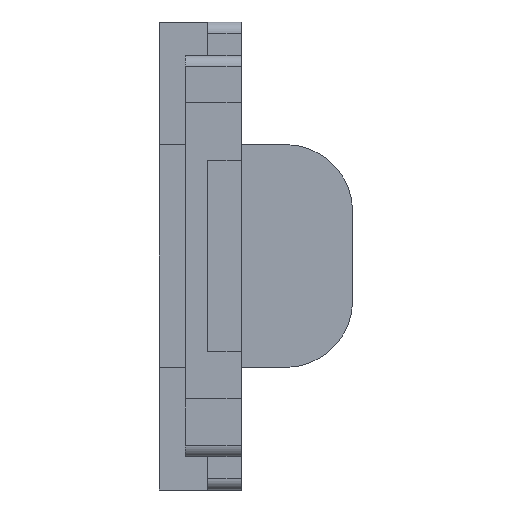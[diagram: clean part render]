
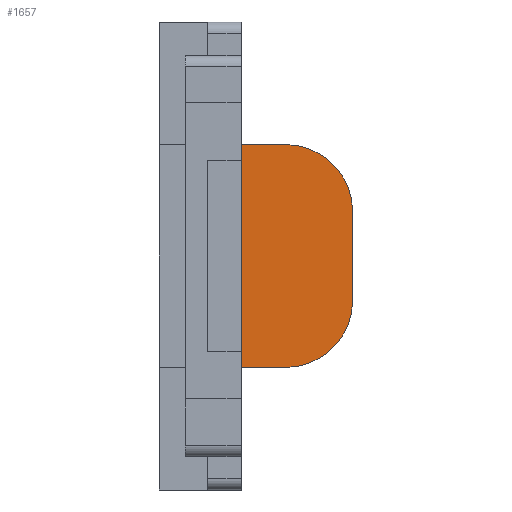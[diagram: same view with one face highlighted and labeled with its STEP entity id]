
A CAD part, front view. The second image highlights one B-rep face of the part: STEP entity #1657.
In plain terms, the highlighted planar face has unit normal (0, -1, 0).
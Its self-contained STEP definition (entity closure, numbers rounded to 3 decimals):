
#162 = PLANE('',#163);
#163 = AXIS2_PLACEMENT_3D('',#164,#165,#166);
#164 = CARTESIAN_POINT('',(8.,-4.,20.));
#165 = DIRECTION('',(1.,0.,0.));
#166 = DIRECTION('',(0.,0.,-1.));
#179 = VERTEX_POINT('',#180);
#180 = CARTESIAN_POINT('',(8.,-4.,20.));
#514 = PLANE('',#515);
#515 = AXIS2_PLACEMENT_3D('',#516,#517,#518);
#516 = CARTESIAN_POINT('',(0.,0.,20.));
#517 = DIRECTION('',(0.,0.,1.));
#518 = DIRECTION('',(1.,0.,0.));
#795 = VERTEX_POINT('',#796);
#796 = CARTESIAN_POINT('',(8.,-4.,0.));
#817 = EDGE_CURVE('',#795,#179,#818,.T.);
#818 = SURFACE_CURVE('',#819,(#823,#830),.PCURVE_S1.);
#819 = LINE('',#820,#821);
#820 = CARTESIAN_POINT('',(8.,-4.,-11.));
#821 = VECTOR('',#822,1.);
#822 = DIRECTION('',(0.,0.,1.));
#823 = PCURVE('',#162,#824);
#824 = DEFINITIONAL_REPRESENTATION('',(#825),#829);
#825 = LINE('',#826,#827);
#826 = CARTESIAN_POINT('',(31.,0.));
#827 = VECTOR('',#828,1.);
#828 = DIRECTION('',(-1.,0.));
#829 = ( GEOMETRIC_REPRESENTATION_CONTEXT(2) 
PARAMETRIC_REPRESENTATION_CONTEXT() REPRESENTATION_CONTEXT('2D SPACE',''
  ) );
#830 = PCURVE('',#831,#836);
#831 = PLANE('',#832);
#832 = AXIS2_PLACEMENT_3D('',#833,#834,#835);
#833 = CARTESIAN_POINT('',(3.,-4.,20.));
#834 = DIRECTION('',(0.,-1.,0.));
#835 = DIRECTION('',(1.,0.,0.));
#836 = DEFINITIONAL_REPRESENTATION('',(#837),#841);
#837 = LINE('',#838,#839);
#838 = CARTESIAN_POINT('',(5.,-31.));
#839 = VECTOR('',#840,1.);
#840 = DIRECTION('',(0.,1.));
#841 = ( GEOMETRIC_REPRESENTATION_CONTEXT(2) 
PARAMETRIC_REPRESENTATION_CONTEXT() REPRESENTATION_CONTEXT('2D SPACE',''
  ) );
#1479 = VERTEX_POINT('',#1480);
#1480 = CARTESIAN_POINT('',(12.,-4.,20.));
#1494 = CYLINDRICAL_SURFACE('',#1495,6.);
#1495 = AXIS2_PLACEMENT_3D('',#1496,#1497,#1498);
#1496 = CARTESIAN_POINT('',(12.,0.,14.));
#1497 = DIRECTION('',(0.,-1.,0.));
#1498 = DIRECTION('',(1.,0.,0.));
#1560 = EDGE_CURVE('',#179,#1479,#1561,.T.);
#1561 = SURFACE_CURVE('',#1562,(#1566,#1573),.PCURVE_S1.);
#1562 = LINE('',#1563,#1564);
#1563 = CARTESIAN_POINT('',(3.,-4.,20.));
#1564 = VECTOR('',#1565,1.);
#1565 = DIRECTION('',(1.,0.,0.));
#1566 = PCURVE('',#514,#1567);
#1567 = DEFINITIONAL_REPRESENTATION('',(#1568),#1572);
#1568 = LINE('',#1569,#1570);
#1569 = CARTESIAN_POINT('',(3.,-4.));
#1570 = VECTOR('',#1571,1.);
#1571 = DIRECTION('',(1.,0.));
#1572 = ( GEOMETRIC_REPRESENTATION_CONTEXT(2) 
PARAMETRIC_REPRESENTATION_CONTEXT() REPRESENTATION_CONTEXT('2D SPACE',''
  ) );
#1573 = PCURVE('',#831,#1574);
#1574 = DEFINITIONAL_REPRESENTATION('',(#1575),#1579);
#1575 = LINE('',#1576,#1577);
#1576 = CARTESIAN_POINT('',(0.,0.));
#1577 = VECTOR('',#1578,1.);
#1578 = DIRECTION('',(1.,0.));
#1579 = ( GEOMETRIC_REPRESENTATION_CONTEXT(2) 
PARAMETRIC_REPRESENTATION_CONTEXT() REPRESENTATION_CONTEXT('2D SPACE',''
  ) );
#1657 = ADVANCED_FACE('',(#1658),#831,.T.);
#1658 = FACE_BOUND('',#1659,.T.);
#1659 = EDGE_LOOP('',(#1660,#1695,#1721,#1743,#1744,#1745));
#1660 = ORIENTED_EDGE('',*,*,#1661,.F.);
#1661 = EDGE_CURVE('',#1662,#1664,#1666,.T.);
#1662 = VERTEX_POINT('',#1663);
#1663 = CARTESIAN_POINT('',(18.,-4.,6.));
#1664 = VERTEX_POINT('',#1665);
#1665 = CARTESIAN_POINT('',(12.,-4.,0.));
#1666 = SURFACE_CURVE('',#1667,(#1672,#1683),.PCURVE_S1.);
#1667 = CIRCLE('',#1668,6.);
#1668 = AXIS2_PLACEMENT_3D('',#1669,#1670,#1671);
#1669 = CARTESIAN_POINT('',(12.,-4.,6.));
#1670 = DIRECTION('',(0.,1.,0.));
#1671 = DIRECTION('',(0.,0.,-1.));
#1672 = PCURVE('',#831,#1673);
#1673 = DEFINITIONAL_REPRESENTATION('',(#1674),#1682);
#1674 = ( BOUNDED_CURVE() B_SPLINE_CURVE(2,(#1675,#1676,#1677,#1678,
#1679,#1680,#1681),.UNSPECIFIED.,.T.,.F.) B_SPLINE_CURVE_WITH_KNOTS((1,2
    ,2,2,2,1),(-2.094,0.,2.094,4.189,
6.283,8.378),.UNSPECIFIED.) CURVE() 
GEOMETRIC_REPRESENTATION_ITEM() RATIONAL_B_SPLINE_CURVE((1.,0.5,1.,0.5,
1.,0.5,1.)) REPRESENTATION_ITEM('') );
#1675 = CARTESIAN_POINT('',(9.,-20.));
#1676 = CARTESIAN_POINT('',(-1.392,-20.));
#1677 = CARTESIAN_POINT('',(3.804,-11.));
#1678 = CARTESIAN_POINT('',(9.,-2.));
#1679 = CARTESIAN_POINT('',(14.196,-11.));
#1680 = CARTESIAN_POINT('',(19.392,-20.));
#1681 = CARTESIAN_POINT('',(9.,-20.));
#1682 = ( GEOMETRIC_REPRESENTATION_CONTEXT(2) 
PARAMETRIC_REPRESENTATION_CONTEXT() REPRESENTATION_CONTEXT('2D SPACE',''
  ) );
#1683 = PCURVE('',#1684,#1689);
#1684 = CYLINDRICAL_SURFACE('',#1685,6.);
#1685 = AXIS2_PLACEMENT_3D('',#1686,#1687,#1688);
#1686 = CARTESIAN_POINT('',(12.,0.,6.));
#1687 = DIRECTION('',(0.,-1.,0.));
#1688 = DIRECTION('',(1.,0.,0.));
#1689 = DEFINITIONAL_REPRESENTATION('',(#1690),#1694);
#1690 = LINE('',#1691,#1692);
#1691 = CARTESIAN_POINT('',(4.712,4.));
#1692 = VECTOR('',#1693,1.);
#1693 = DIRECTION('',(-1.,0.));
#1694 = ( GEOMETRIC_REPRESENTATION_CONTEXT(2) 
PARAMETRIC_REPRESENTATION_CONTEXT() REPRESENTATION_CONTEXT('2D SPACE',''
  ) );
#1695 = ORIENTED_EDGE('',*,*,#1696,.F.);
#1696 = EDGE_CURVE('',#1697,#1662,#1699,.T.);
#1697 = VERTEX_POINT('',#1698);
#1698 = CARTESIAN_POINT('',(18.,-4.,14.));
#1699 = SURFACE_CURVE('',#1700,(#1704,#1710),.PCURVE_S1.);
#1700 = LINE('',#1701,#1702);
#1701 = CARTESIAN_POINT('',(18.,-4.,10.));
#1702 = VECTOR('',#1703,1.);
#1703 = DIRECTION('',(0.,0.,-1.));
#1704 = PCURVE('',#831,#1705);
#1705 = DEFINITIONAL_REPRESENTATION('',(#1706),#1709);
#1706 = B_SPLINE_CURVE_WITH_KNOTS('',1,(#1707,#1708),.UNSPECIFIED.,.F.,
  .F.,(2,2),(-12.,12.),.PIECEWISE_BEZIER_KNOTS.);
#1707 = CARTESIAN_POINT('',(15.,2.));
#1708 = CARTESIAN_POINT('',(15.,-22.));
#1709 = ( GEOMETRIC_REPRESENTATION_CONTEXT(2) 
PARAMETRIC_REPRESENTATION_CONTEXT() REPRESENTATION_CONTEXT('2D SPACE',''
  ) );
#1710 = PCURVE('',#1711,#1716);
#1711 = PLANE('',#1712);
#1712 = AXIS2_PLACEMENT_3D('',#1713,#1714,#1715);
#1713 = CARTESIAN_POINT('',(18.,0.,0.));
#1714 = DIRECTION('',(1.,0.,0.));
#1715 = DIRECTION('',(0.,-1.,0.));
#1716 = DEFINITIONAL_REPRESENTATION('',(#1717),#1720);
#1717 = B_SPLINE_CURVE_WITH_KNOTS('',1,(#1718,#1719),.UNSPECIFIED.,.F.,
  .F.,(2,2),(-12.,12.),.PIECEWISE_BEZIER_KNOTS.);
#1718 = CARTESIAN_POINT('',(4.,-22.));
#1719 = CARTESIAN_POINT('',(4.,2.));
#1720 = ( GEOMETRIC_REPRESENTATION_CONTEXT(2) 
PARAMETRIC_REPRESENTATION_CONTEXT() REPRESENTATION_CONTEXT('2D SPACE',''
  ) );
#1721 = ORIENTED_EDGE('',*,*,#1722,.T.);
#1722 = EDGE_CURVE('',#1697,#1479,#1723,.T.);
#1723 = SURFACE_CURVE('',#1724,(#1729,#1736),.PCURVE_S1.);
#1724 = CIRCLE('',#1725,6.);
#1725 = AXIS2_PLACEMENT_3D('',#1726,#1727,#1728);
#1726 = CARTESIAN_POINT('',(12.,-4.,14.));
#1727 = DIRECTION('',(0.,-1.,0.));
#1728 = DIRECTION('',(0.,0.,-1.));
#1729 = PCURVE('',#831,#1730);
#1730 = DEFINITIONAL_REPRESENTATION('',(#1731),#1735);
#1731 = CIRCLE('',#1732,6.);
#1732 = AXIS2_PLACEMENT_2D('',#1733,#1734);
#1733 = CARTESIAN_POINT('',(9.,-6.));
#1734 = DIRECTION('',(0.,-1.));
#1735 = ( GEOMETRIC_REPRESENTATION_CONTEXT(2) 
PARAMETRIC_REPRESENTATION_CONTEXT() REPRESENTATION_CONTEXT('2D SPACE',''
  ) );
#1736 = PCURVE('',#1494,#1737);
#1737 = DEFINITIONAL_REPRESENTATION('',(#1738),#1742);
#1738 = LINE('',#1739,#1740);
#1739 = CARTESIAN_POINT('',(-1.571,4.));
#1740 = VECTOR('',#1741,1.);
#1741 = DIRECTION('',(1.,0.));
#1742 = ( GEOMETRIC_REPRESENTATION_CONTEXT(2) 
PARAMETRIC_REPRESENTATION_CONTEXT() REPRESENTATION_CONTEXT('2D SPACE',''
  ) );
#1743 = ORIENTED_EDGE('',*,*,#1560,.F.);
#1744 = ORIENTED_EDGE('',*,*,#817,.F.);
#1745 = ORIENTED_EDGE('',*,*,#1746,.T.);
#1746 = EDGE_CURVE('',#795,#1664,#1747,.T.);
#1747 = SURFACE_CURVE('',#1748,(#1752,#1758),.PCURVE_S1.);
#1748 = LINE('',#1749,#1750);
#1749 = CARTESIAN_POINT('',(1.5,-4.,0.));
#1750 = VECTOR('',#1751,1.);
#1751 = DIRECTION('',(1.,0.,0.));
#1752 = PCURVE('',#831,#1753);
#1753 = DEFINITIONAL_REPRESENTATION('',(#1754),#1757);
#1754 = B_SPLINE_CURVE_WITH_KNOTS('',1,(#1755,#1756),.UNSPECIFIED.,.F.,
  .F.,(2,2),(-0.816,18.3),.PIECEWISE_BEZIER_KNOTS.);
#1755 = CARTESIAN_POINT('',(-2.316,-20.));
#1756 = CARTESIAN_POINT('',(16.8,-20.));
#1757 = ( GEOMETRIC_REPRESENTATION_CONTEXT(2) 
PARAMETRIC_REPRESENTATION_CONTEXT() REPRESENTATION_CONTEXT('2D SPACE',''
  ) );
#1758 = PCURVE('',#1759,#1764);
#1759 = PLANE('',#1760);
#1760 = AXIS2_PLACEMENT_3D('',#1761,#1762,#1763);
#1761 = CARTESIAN_POINT('',(0.,0.,0.));
#1762 = DIRECTION('',(0.,0.,1.));
#1763 = DIRECTION('',(1.,0.,0.));
#1764 = DEFINITIONAL_REPRESENTATION('',(#1765),#1768);
#1765 = B_SPLINE_CURVE_WITH_KNOTS('',1,(#1766,#1767),.UNSPECIFIED.,.F.,
  .F.,(2,2),(-0.816,18.3),.PIECEWISE_BEZIER_KNOTS.);
#1766 = CARTESIAN_POINT('',(0.684,-4.));
#1767 = CARTESIAN_POINT('',(19.8,-4.));
#1768 = ( GEOMETRIC_REPRESENTATION_CONTEXT(2) 
PARAMETRIC_REPRESENTATION_CONTEXT() REPRESENTATION_CONTEXT('2D SPACE',''
  ) );
